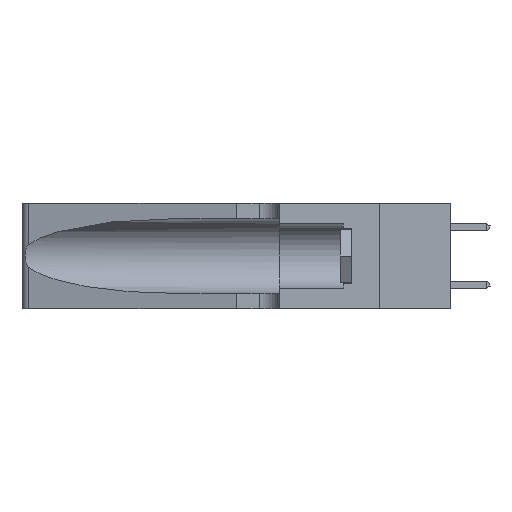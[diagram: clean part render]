
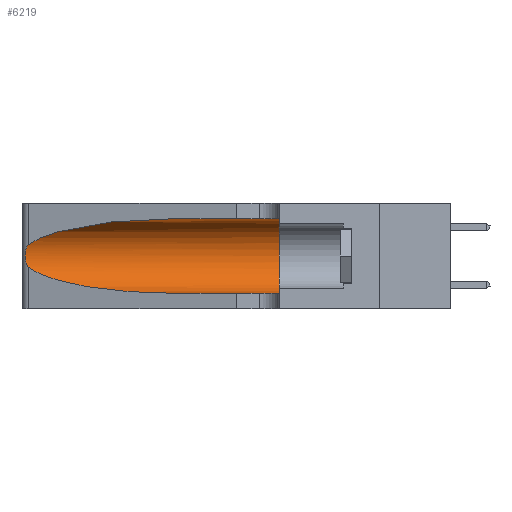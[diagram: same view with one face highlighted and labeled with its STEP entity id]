
A CAD part, left-side view. The second image highlights one B-rep face of the part: STEP entity #6219.
In plain terms, the highlighted cylindrical face has radius 3.308 mm (diameter 6.617 mm), a partial arc.
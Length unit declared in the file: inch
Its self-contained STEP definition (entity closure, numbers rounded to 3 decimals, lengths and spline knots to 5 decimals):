
#195 = CARTESIAN_POINT ( 'NONE',  ( 0.2373, 1.15595, 0.08982 ) ) ;
#266 = EDGE_CURVE ( 'NONE', #22823, #11970, #30161, .T. ) ;
#336 = ORIENTED_EDGE ( 'NONE', *, *, #20127, .T. ) ;
#341 = LINE ( 'NONE', #3714, #28547 ) ;
#1211 = CARTESIAN_POINT ( 'NONE',  ( 0.25487, 1.22718, 0.14631 ) ) ;
#1530 = VERTEX_POINT ( 'NONE', #4942 ) ;
#1827 = CARTESIAN_POINT ( 'NONE',  ( 0.26075, 1.23896, 0.19203 ) ) ;
#2895 =( BOUNDED_CURVE ( )  B_SPLINE_CURVE ( 3, ( #5918, #195, #31200, #14450 ),
 .UNSPECIFIED., .F., .T. ) 
 B_SPLINE_CURVE_WITH_KNOTS ( ( 4, 4 ),
 ( 3.44316, 4.71239 ),
 .UNSPECIFIED. ) 
 CURVE ( )  GEOMETRIC_REPRESENTATION_ITEM ( )  RATIONAL_B_SPLINE_CURVE ( ( 1., 0.87, 0.87, 1. ) ) 
 REPRESENTATION_ITEM ( '' )  );
#3549 = LINE ( 'NONE', #27967, #10220 ) ;
#3714 = CARTESIAN_POINT ( 'NONE',  ( 0.1305, 1.61858, 0.31525 ) ) ;
#4079 = CARTESIAN_POINT ( 'NONE',  ( 0.1305, 0.35, 0.31525 ) ) ;
#4323 = FACE_OUTER_BOUND ( 'NONE', #31894, .T. ) ;
#4697 = CARTESIAN_POINT ( 'NONE',  ( 0.26017, 1.23833, 0.17102 ) ) ;
#4942 = CARTESIAN_POINT ( 'NONE',  ( 0.25487, 1.22718, 0.22369 ) ) ;
#5918 = CARTESIAN_POINT ( 'NONE',  ( 0.25487, 1.22718, 0.14631 ) ) ;
#6113 = CARTESIAN_POINT ( 'NONE',  ( 0.1305, 0.72297, 0.31525 ) ) ;
#6219 = ADVANCED_FACE ( 'NONE', ( #4323 ), #18430, .F. ) ;
#7131 = CARTESIAN_POINT ( 'NONE',  ( 0.1305, 0.72297, 0.31525 ) ) ;
#8036 = CARTESIAN_POINT ( 'NONE',  ( 0.25789, 1.23486, 0.15765 ) ) ;
#8159 = AXIS2_PLACEMENT_3D ( 'NONE', #33513, #25069, #30690 ) ;
#8876 = CARTESIAN_POINT ( 'NONE',  ( 0.1305, 0.72297, 0.05475 ) ) ;
#8897 = VERTEX_POINT ( 'NONE', #8876 ) ;
#10220 = VECTOR ( 'NONE', #30775, 39.37008 ) ;
#10876 = CARTESIAN_POINT ( 'NONE',  ( 0.25555, 1.22993, 0.14849 ) ) ;
#11788 = CARTESIAN_POINT ( 'NONE',  ( 0.2373, 1.15595, 0.28018 ) ) ;
#11970 = VERTEX_POINT ( 'NONE', #33028 ) ;
#12987 = VERTEX_POINT ( 'NONE', #1211 ) ;
#13107 = CARTESIAN_POINT ( 'NONE',  ( 0.25555, 1.22994, 0.2215 ) ) ;
#14450 = CARTESIAN_POINT ( 'NONE',  ( 0.1305, 0.72297, 0.05475 ) ) ;
#15928 = CARTESIAN_POINT ( 'NONE',  ( 0.25787, 1.23484, 0.2124 ) ) ;
#15948 = EDGE_CURVE ( 'NONE', #33294, #1530, #22540, .T. ) ;
#16705 = CARTESIAN_POINT ( 'NONE',  ( 0.1305, 0.35, 0.185 ) ) ;
#17170 = ORIENTED_EDGE ( 'NONE', *, *, #19590, .F. ) ;
#18326 = EDGE_CURVE ( 'NONE', #8897, #11970, #3549, .T. ) ;
#18430 = CYLINDRICAL_SURFACE ( 'NONE', #8159, 0.13025 ) ;
#18735 = CARTESIAN_POINT ( 'NONE',  ( 0.26018, 1.23835, 0.19895 ) ) ;
#19590 = EDGE_CURVE ( 'NONE', #33294, #22823, #341, .T. ) ;
#20127 = EDGE_CURVE ( 'NONE', #12987, #8897, #2895, .T. ) ;
#20228 = ORIENTED_EDGE ( 'NONE', *, *, #15948, .T. ) ;
#20595 = DIRECTION ( 'NONE',  ( 0., -1., 0. ) ) ;
#21423 = CARTESIAN_POINT ( 'NONE',  ( 0.25487, 1.22718, 0.22369 ) ) ;
#21538 = CARTESIAN_POINT ( 'NONE',  ( 0.26075, 1.23896, 0.178 ) ) ;
#21979 = ORIENTED_EDGE ( 'NONE', *, *, #24946, .T. ) ;
#22540 =( BOUNDED_CURVE ( )  B_SPLINE_CURVE ( 3, ( #6113, #22946, #11788, #31389 ),
 .UNSPECIFIED., .F., .T. ) 
 B_SPLINE_CURVE_WITH_KNOTS ( ( 4, 4 ),
 ( 1.5708, 2.84003 ),
 .UNSPECIFIED. ) 
 CURVE ( )  GEOMETRIC_REPRESENTATION_ITEM ( )  RATIONAL_B_SPLINE_CURVE ( ( 1., 0.87, 0.87, 1. ) ) 
 REPRESENTATION_ITEM ( '' )  );
#22823 = VERTEX_POINT ( 'NONE', #4079 ) ;
#22946 = CARTESIAN_POINT ( 'NONE',  ( 0.18966, 0.96281, 0.31525 ) ) ;
#23723 = ORIENTED_EDGE ( 'NONE', *, *, #18326, .T. ) ;
#24860 = CARTESIAN_POINT ( 'NONE',  ( 0.25856, 1.23593, 0.16098 ) ) ;
#24946 = EDGE_CURVE ( 'NONE', #1530, #12987, #26350, .T. ) ;
#25069 = DIRECTION ( 'NONE',  ( 0., -1., 0. ) ) ;
#26350 = B_SPLINE_CURVE_WITH_KNOTS ( 'NONE', 3,
 ( #21423, #13107, #32691, #15928, #35513, #18735, #1827, #21538, #4697, #24860, #8036, #27681, #10876, #30481 ),
 .UNSPECIFIED., .F., .F.,
 ( 4, 2, 2, 2, 2, 2, 4 ),
 ( 0., 0.00027, 0.00053, 0.00107, 0.0016, 0.00187, 0.00214 ),
 .UNSPECIFIED. ) ;
#27681 = CARTESIAN_POINT ( 'NONE',  ( 0.25639, 1.23186, 0.15144 ) ) ;
#27967 = CARTESIAN_POINT ( 'NONE',  ( 0.1305, 1.61858, 0.05475 ) ) ;
#28547 = VECTOR ( 'NONE', #20595, 39.37008 ) ;
#30161 = CIRCLE ( 'NONE', #35794, 0.13025 ) ;
#30481 = CARTESIAN_POINT ( 'NONE',  ( 0.25487, 1.22718, 0.14631 ) ) ;
#30690 = DIRECTION ( 'NONE',  ( 0., 0., -1. ) ) ;
#30775 = DIRECTION ( 'NONE',  ( 0., -1., 0. ) ) ;
#31172 = ORIENTED_EDGE ( 'NONE', *, *, #266, .F. ) ;
#31200 = CARTESIAN_POINT ( 'NONE',  ( 0.18966, 0.96281, 0.05475 ) ) ;
#31389 = CARTESIAN_POINT ( 'NONE',  ( 0.25487, 1.22718, 0.22369 ) ) ;
#31894 = EDGE_LOOP ( 'NONE', ( #20228, #21979, #336, #23723, #31172, #17170 ) ) ;
#32691 = CARTESIAN_POINT ( 'NONE',  ( 0.25639, 1.23184, 0.21858 ) ) ;
#33028 = CARTESIAN_POINT ( 'NONE',  ( 0.1305, 0.35, 0.05475 ) ) ;
#33294 = VERTEX_POINT ( 'NONE', #7131 ) ;
#33425 = DIRECTION ( 'NONE',  ( 0., 1., 0. ) ) ;
#33513 = CARTESIAN_POINT ( 'NONE',  ( 0.1305, 1.61858, 0.185 ) ) ;
#34502 = DIRECTION ( 'NONE',  ( 0., 0., 1. ) ) ;
#35513 = CARTESIAN_POINT ( 'NONE',  ( 0.25854, 1.2359, 0.20912 ) ) ;
#35794 = AXIS2_PLACEMENT_3D ( 'NONE', #16705, #33425, #34502 ) ;
